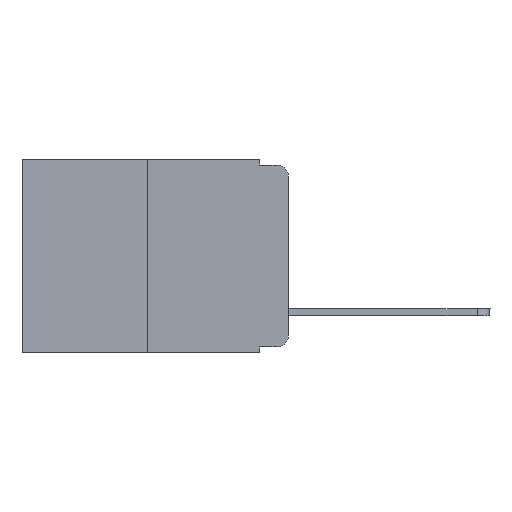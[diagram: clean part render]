
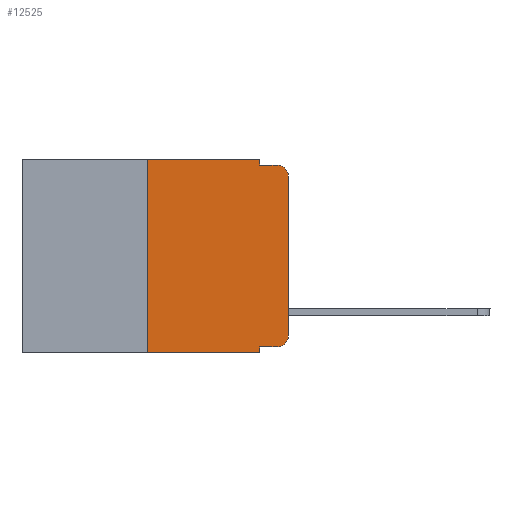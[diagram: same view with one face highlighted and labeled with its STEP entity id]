
A CAD part, left-side view. The second image highlights one B-rep face of the part: STEP entity #12525.
In plain terms, the highlighted planar face has unit normal (-1, 0, 0).
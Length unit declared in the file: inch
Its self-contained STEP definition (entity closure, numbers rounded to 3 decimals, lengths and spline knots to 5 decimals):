
#182 = EDGE_CURVE ( 'NONE', #13425, #1206, #1586, .T. ) ;
#379 = DIRECTION ( 'NONE',  ( -1., 0., 0. ) ) ;
#725 = VECTOR ( 'NONE', #10988, 39.37008 ) ;
#1094 = CARTESIAN_POINT ( 'NONE',  ( 0., 0., 0. ) ) ;
#1206 = VERTEX_POINT ( 'NONE', #8907 ) ;
#1336 = DIRECTION ( 'NONE',  ( 0., 0., -1. ) ) ;
#1394 = VECTOR ( 'NONE', #7478, 39.37008 ) ;
#1490 = LINE ( 'NONE', #13578, #725 ) ;
#1586 = CIRCLE ( 'NONE', #12800, 0.02 ) ;
#1650 = DIRECTION ( 'NONE',  ( 0., 0., -1. ) ) ;
#1800 = EDGE_CURVE ( 'NONE', #15169, #11039, #3962, .T. ) ;
#2302 = CARTESIAN_POINT ( 'NONE',  ( 0., 0.051, 0. ) ) ;
#2801 = CARTESIAN_POINT ( 'NONE',  ( 0., 0.25, -0.343 ) ) ;
#3020 = ORIENTED_EDGE ( 'NONE', *, *, #15197, .F. ) ;
#3130 = VERTEX_POINT ( 'NONE', #2302 ) ;
#3311 = DIRECTION ( 'NONE',  ( 0., -1., 0. ) ) ;
#3411 = CARTESIAN_POINT ( 'NONE',  ( 0., 0.02, -0.333 ) ) ;
#3413 = FACE_OUTER_BOUND ( 'NONE', #6764, .T. ) ;
#3417 = ORIENTED_EDGE ( 'NONE', *, *, #10029, .F. ) ;
#3692 = VECTOR ( 'NONE', #1336, 39.37008 ) ;
#3962 = LINE ( 'NONE', #7705, #1394 ) ;
#4295 = CIRCLE ( 'NONE', #4546, 0.02 ) ;
#4546 = AXIS2_PLACEMENT_3D ( 'NONE', #12410, #10144, #1650 ) ;
#4672 = DIRECTION ( 'NONE',  ( 1., 0., 0. ) ) ;
#4790 = VERTEX_POINT ( 'NONE', #13799 ) ;
#5091 = EDGE_CURVE ( 'NONE', #11269, #9577, #4295, .T. ) ;
#5146 = LINE ( 'NONE', #14579, #14226 ) ;
#5233 = ORIENTED_EDGE ( 'NONE', *, *, #9301, .T. ) ;
#5428 = AXIS2_PLACEMENT_3D ( 'NONE', #13084, #4672, #10737 ) ;
#5727 = VECTOR ( 'NONE', #3311, 39.37008 ) ;
#5837 = PLANE ( 'NONE',  #5428 ) ;
#5910 = ORIENTED_EDGE ( 'NONE', *, *, #11186, .F. ) ;
#5915 = ORIENTED_EDGE ( 'NONE', *, *, #5091, .T. ) ;
#6764 = EDGE_LOOP ( 'NONE', ( #5233, #14891, #3417, #14261, #3020, #11005, #11543, #5910, #12749, #5915 ) ) ;
#7034 = LINE ( 'NONE', #1094, #14244 ) ;
#7416 = VECTOR ( 'NONE', #15391, 39.37008 ) ;
#7478 = DIRECTION ( 'NONE',  ( 0., -1., 0. ) ) ;
#7494 = CARTESIAN_POINT ( 'NONE',  ( 0., 0.02, -0.03 ) ) ;
#7705 = CARTESIAN_POINT ( 'NONE',  ( 0., 0.473, -0.343 ) ) ;
#7765 = EDGE_CURVE ( 'NONE', #15169, #4790, #5146, .T. ) ;
#8671 = CARTESIAN_POINT ( 'NONE',  ( 0., 0.051, -0.333 ) ) ;
#8875 = CARTESIAN_POINT ( 'NONE',  ( 0., 0.051, -0.01 ) ) ;
#8907 = CARTESIAN_POINT ( 'NONE',  ( 0., 0.02, -0.01 ) ) ;
#9301 = EDGE_CURVE ( 'NONE', #9577, #13425, #7034, .T. ) ;
#9345 = LINE ( 'NONE', #14228, #3692 ) ;
#9577 = VERTEX_POINT ( 'NONE', #12688 ) ;
#9668 = LINE ( 'NONE', #13207, #7416 ) ;
#10029 = EDGE_CURVE ( 'NONE', #10557, #1206, #11409, .T. ) ;
#10144 = DIRECTION ( 'NONE',  ( -1., 0., 0. ) ) ;
#10200 = LINE ( 'NONE', #13644, #14002 ) ;
#10557 = VERTEX_POINT ( 'NONE', #8875 ) ;
#10737 = DIRECTION ( 'NONE',  ( 0., 0., -1. ) ) ;
#10988 = DIRECTION ( 'NONE',  ( 0., -1., 0. ) ) ;
#11005 = ORIENTED_EDGE ( 'NONE', *, *, #7765, .F. ) ;
#11039 = VERTEX_POINT ( 'NONE', #14658 ) ;
#11186 = EDGE_CURVE ( 'NONE', #14386, #11039, #10200, .T. ) ;
#11269 = VERTEX_POINT ( 'NONE', #3411 ) ;
#11331 = CARTESIAN_POINT ( 'NONE',  ( 0., 0.051, -0.01 ) ) ;
#11409 = LINE ( 'NONE', #11331, #5727 ) ;
#11447 = DIRECTION ( 'NONE',  ( 0., 0., -1. ) ) ;
#11543 = ORIENTED_EDGE ( 'NONE', *, *, #1800, .T. ) ;
#11546 = DIRECTION ( 'NONE',  ( 0., 0., 1. ) ) ;
#12410 = CARTESIAN_POINT ( 'NONE',  ( 0., 0.02, -0.313 ) ) ;
#12482 = DIRECTION ( 'NONE',  ( 0., 0., -1. ) ) ;
#12525 = ADVANCED_FACE ( 'NONE', ( #3413 ), #5837, .F. ) ;
#12688 = CARTESIAN_POINT ( 'NONE',  ( 0., 0., -0.313 ) ) ;
#12749 = ORIENTED_EDGE ( 'NONE', *, *, #14534, .T. ) ;
#12800 = AXIS2_PLACEMENT_3D ( 'NONE', #7494, #379, #12482 ) ;
#13084 = CARTESIAN_POINT ( 'NONE',  ( 0., 0.473, 0. ) ) ;
#13207 = CARTESIAN_POINT ( 'NONE',  ( 0., 0.051, -0.333 ) ) ;
#13425 = VERTEX_POINT ( 'NONE', #14088 ) ;
#13568 = DIRECTION ( 'NONE',  ( 0., 0., 1. ) ) ;
#13578 = CARTESIAN_POINT ( 'NONE',  ( 0., 0.473, 0. ) ) ;
#13644 = CARTESIAN_POINT ( 'NONE',  ( 0., 0.051, 0. ) ) ;
#13799 = CARTESIAN_POINT ( 'NONE',  ( 0., 0.25, 0. ) ) ;
#14002 = VECTOR ( 'NONE', #11447, 39.37008 ) ;
#14088 = CARTESIAN_POINT ( 'NONE',  ( 0., 0., -0.03 ) ) ;
#14226 = VECTOR ( 'NONE', #13568, 39.37008 ) ;
#14228 = CARTESIAN_POINT ( 'NONE',  ( 0., 0.051, 0. ) ) ;
#14244 = VECTOR ( 'NONE', #11546, 39.37008 ) ;
#14261 = ORIENTED_EDGE ( 'NONE', *, *, #14949, .F. ) ;
#14386 = VERTEX_POINT ( 'NONE', #8671 ) ;
#14534 = EDGE_CURVE ( 'NONE', #14386, #11269, #9668, .T. ) ;
#14579 = CARTESIAN_POINT ( 'NONE',  ( 0., 0.25, 0. ) ) ;
#14658 = CARTESIAN_POINT ( 'NONE',  ( 0., 0.051, -0.343 ) ) ;
#14891 = ORIENTED_EDGE ( 'NONE', *, *, #182, .T. ) ;
#14949 = EDGE_CURVE ( 'NONE', #3130, #10557, #9345, .T. ) ;
#15169 = VERTEX_POINT ( 'NONE', #2801 ) ;
#15197 = EDGE_CURVE ( 'NONE', #4790, #3130, #1490, .T. ) ;
#15391 = DIRECTION ( 'NONE',  ( 0., -1., 0. ) ) ;
